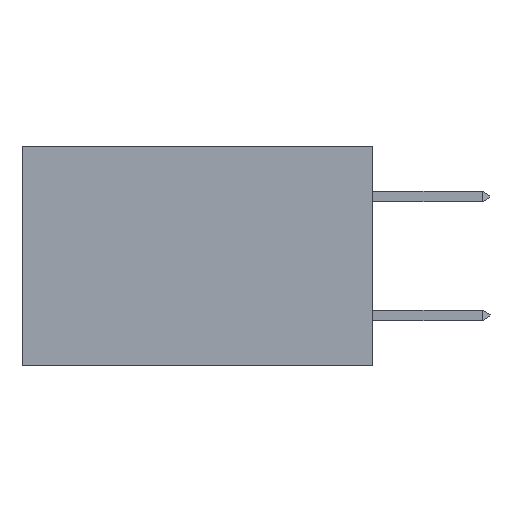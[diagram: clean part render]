
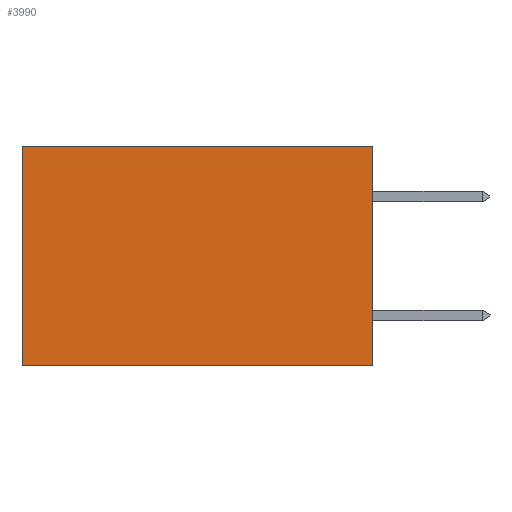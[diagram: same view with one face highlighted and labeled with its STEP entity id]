
A CAD part, left-side view. The second image highlights one B-rep face of the part: STEP entity #3990.
In plain terms, the highlighted planar face has unit normal (-1, 0, 0).
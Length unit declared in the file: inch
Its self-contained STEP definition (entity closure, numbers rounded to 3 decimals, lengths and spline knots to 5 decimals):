
#458 = CARTESIAN_POINT ( 'NONE',  ( 0.277, 0.59, -0.37 ) ) ;
#923 = EDGE_CURVE ( 'NONE', #4423, #5482, #6357, .T. ) ;
#1097 = EDGE_CURVE ( 'NONE', #10218, #4423, #14291, .T. ) ;
#1519 = EDGE_CURVE ( 'NONE', #10218, #6131, #4704, .T. ) ;
#1603 = CARTESIAN_POINT ( 'NONE',  ( 0.277, 0., -0.37 ) ) ;
#1828 = ORIENTED_EDGE ( 'NONE', *, *, #1519, .F. ) ;
#2834 = VECTOR ( 'NONE', #4947, 39.37008 ) ;
#3691 = ORIENTED_EDGE ( 'NONE', *, *, #923, .T. ) ;
#3990 = ADVANCED_FACE ( 'NONE', ( #15210 ), #5222, .F. ) ;
#4052 = CARTESIAN_POINT ( 'NONE',  ( 0.277, 0., 0. ) ) ;
#4303 = VECTOR ( 'NONE', #5488, 39.37008 ) ;
#4423 = VERTEX_POINT ( 'NONE', #15106 ) ;
#4502 = ORIENTED_EDGE ( 'NONE', *, *, #1097, .T. ) ;
#4704 = LINE ( 'NONE', #5315, #14657 ) ;
#4883 = CARTESIAN_POINT ( 'NONE',  ( 0.277, 0., 0. ) ) ;
#4947 = DIRECTION ( 'NONE',  ( 0., 0., -1. ) ) ;
#5222 = PLANE ( 'NONE',  #11724 ) ;
#5315 = CARTESIAN_POINT ( 'NONE',  ( 0.277, 0., -0.37 ) ) ;
#5482 = VERTEX_POINT ( 'NONE', #458 ) ;
#5488 = DIRECTION ( 'NONE',  ( 0., 1., 0. ) ) ;
#5622 = DIRECTION ( 'NONE',  ( 0., 0., -1. ) ) ;
#5629 = LINE ( 'NONE', #7378, #8701 ) ;
#6131 = VERTEX_POINT ( 'NONE', #1603 ) ;
#6357 = LINE ( 'NONE', #13257, #2834 ) ;
#6551 = DIRECTION ( 'NONE',  ( 0., 0., -1. ) ) ;
#7378 = CARTESIAN_POINT ( 'NONE',  ( 0.277, 0., -0.37 ) ) ;
#7996 = ORIENTED_EDGE ( 'NONE', *, *, #16294, .F. ) ;
#8329 = EDGE_LOOP ( 'NONE', ( #3691, #7996, #1828, #4502 ) ) ;
#8701 = VECTOR ( 'NONE', #16441, 39.37008 ) ;
#10218 = VERTEX_POINT ( 'NONE', #4883 ) ;
#11724 = AXIS2_PLACEMENT_3D ( 'NONE', #11735, #14335, #6551 ) ;
#11735 = CARTESIAN_POINT ( 'NONE',  ( 0.277, 0., -0.37 ) ) ;
#13257 = CARTESIAN_POINT ( 'NONE',  ( 0.277, 0.59, -0.37 ) ) ;
#14291 = LINE ( 'NONE', #4052, #4303 ) ;
#14335 = DIRECTION ( 'NONE',  ( 1., 0., 0. ) ) ;
#14657 = VECTOR ( 'NONE', #5622, 39.37008 ) ;
#15106 = CARTESIAN_POINT ( 'NONE',  ( 0.277, 0.59, 0. ) ) ;
#15210 = FACE_OUTER_BOUND ( 'NONE', #8329, .T. ) ;
#16294 = EDGE_CURVE ( 'NONE', #6131, #5482, #5629, .T. ) ;
#16441 = DIRECTION ( 'NONE',  ( 0., 1., 0. ) ) ;
